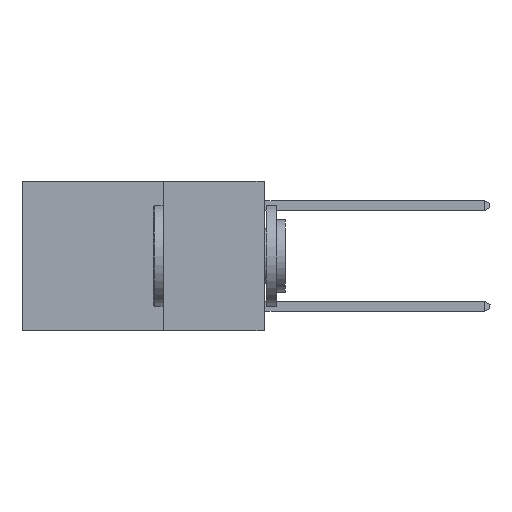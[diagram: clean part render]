
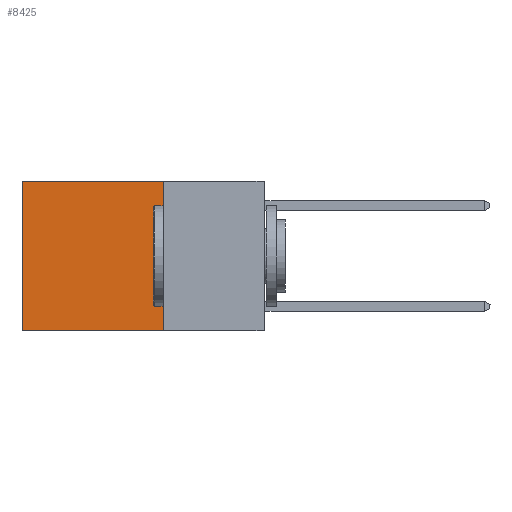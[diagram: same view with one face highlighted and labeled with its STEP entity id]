
A CAD part, left-side view. The second image highlights one B-rep face of the part: STEP entity #8425.
In plain terms, the highlighted planar face has unit normal (-1, 0, 0).
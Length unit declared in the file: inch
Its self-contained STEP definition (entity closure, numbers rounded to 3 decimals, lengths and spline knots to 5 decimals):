
#256 = ORIENTED_EDGE ( 'NONE', *, *, #12296, .F. ) ;
#586 = VERTEX_POINT ( 'NONE', #8132 ) ;
#1147 = VERTEX_POINT ( 'NONE', #9389 ) ;
#1333 = VERTEX_POINT ( 'NONE', #1920 ) ;
#1401 = DIRECTION ( 'NONE',  ( 0., 0., -1. ) ) ;
#1920 = CARTESIAN_POINT ( 'NONE',  ( 0.2625, 0.6, 0. ) ) ;
#1969 = VECTOR ( 'NONE', #16929, 39.37008 ) ;
#2970 = EDGE_CURVE ( 'NONE', #4221, #1147, #16671, .T. ) ;
#3091 = EDGE_CURVE ( 'NONE', #1333, #586, #14203, .T. ) ;
#4221 = VERTEX_POINT ( 'NONE', #9693 ) ;
#4253 = ORIENTED_EDGE ( 'NONE', *, *, #2970, .F. ) ;
#5052 = EDGE_LOOP ( 'NONE', ( #7244, #256, #4253, #10234 ) ) ;
#5611 = CARTESIAN_POINT ( 'NONE',  ( 0.2625, 0.25, 0. ) ) ;
#5997 = DIRECTION ( 'NONE',  ( 0., 1., 0. ) ) ;
#6399 = VECTOR ( 'NONE', #20252, 39.37008 ) ;
#7244 = ORIENTED_EDGE ( 'NONE', *, *, #3091, .T. ) ;
#8132 = CARTESIAN_POINT ( 'NONE',  ( 0.2625, 0.6, -0.37 ) ) ;
#8425 = ADVANCED_FACE ( 'NONE', ( #13443 ), #20215, .F. ) ;
#8628 = VECTOR ( 'NONE', #5997, 39.37008 ) ;
#9155 = CARTESIAN_POINT ( 'NONE',  ( 0.2625, 0.25, -0.37 ) ) ;
#9330 = CARTESIAN_POINT ( 'NONE',  ( 0.2625, 0.6, 0. ) ) ;
#9389 = CARTESIAN_POINT ( 'NONE',  ( 0.2625, 0.25, -0.37 ) ) ;
#9693 = CARTESIAN_POINT ( 'NONE',  ( 0.2625, 0.25, 0. ) ) ;
#10234 = ORIENTED_EDGE ( 'NONE', *, *, #13476, .T. ) ;
#10870 = DIRECTION ( 'NONE',  ( 1., 0., 0. ) ) ;
#11333 = AXIS2_PLACEMENT_3D ( 'NONE', #15496, #10870, #1401 ) ;
#12296 = EDGE_CURVE ( 'NONE', #1147, #586, #18190, .T. ) ;
#12521 = VECTOR ( 'NONE', #18143, 39.37008 ) ;
#13443 = FACE_OUTER_BOUND ( 'NONE', #5052, .T. ) ;
#13476 = EDGE_CURVE ( 'NONE', #4221, #1333, #16428, .T. ) ;
#14203 = LINE ( 'NONE', #9330, #6399 ) ;
#15496 = CARTESIAN_POINT ( 'NONE',  ( 0.2625, 0.25, 0. ) ) ;
#16428 = LINE ( 'NONE', #16942, #8628 ) ;
#16671 = LINE ( 'NONE', #5611, #12521 ) ;
#16929 = DIRECTION ( 'NONE',  ( 0., 1., 0. ) ) ;
#16942 = CARTESIAN_POINT ( 'NONE',  ( 0.2625, 0.25, 0. ) ) ;
#18143 = DIRECTION ( 'NONE',  ( 0., 0., -1. ) ) ;
#18190 = LINE ( 'NONE', #9155, #1969 ) ;
#20215 = PLANE ( 'NONE',  #11333 ) ;
#20252 = DIRECTION ( 'NONE',  ( 0., 0., -1. ) ) ;
